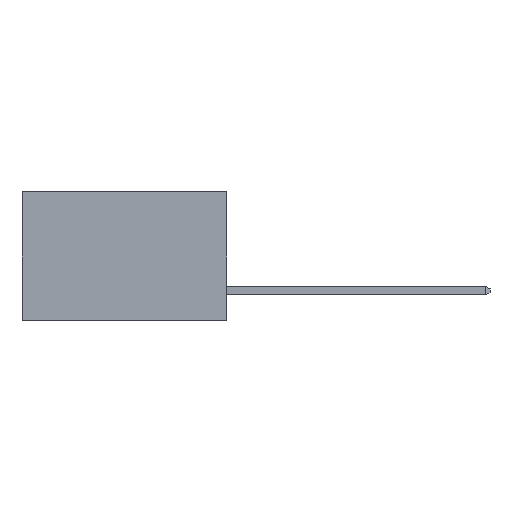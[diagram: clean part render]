
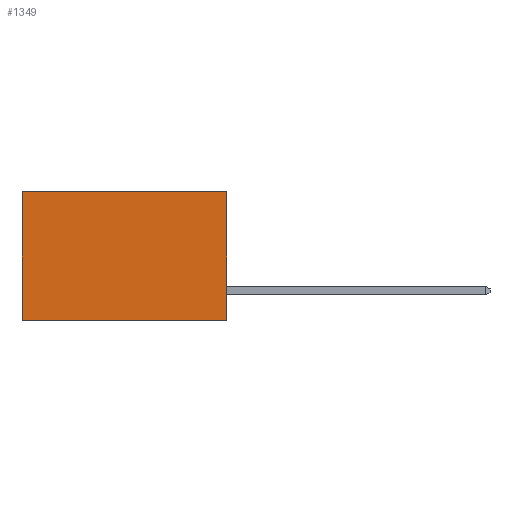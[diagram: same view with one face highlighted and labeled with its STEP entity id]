
A CAD part, left-side view. The second image highlights one B-rep face of the part: STEP entity #1349.
In plain terms, the highlighted planar face has unit normal (-1, 0, 0).
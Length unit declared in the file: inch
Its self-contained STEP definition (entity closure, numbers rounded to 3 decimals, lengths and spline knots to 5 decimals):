
#685 = VERTEX_POINT ( 'NONE', #7083 ) ;
#694 = DIRECTION ( 'NONE',  ( 0., 1., 0. ) ) ;
#1349 = ADVANCED_FACE ( 'NONE', ( #7775 ), #1897, .F. ) ;
#1603 = VERTEX_POINT ( 'NONE', #3541 ) ;
#1897 = PLANE ( 'NONE',  #5435 ) ;
#2203 = VERTEX_POINT ( 'NONE', #6520 ) ;
#2267 = DIRECTION ( 'NONE',  ( 0., 1., 0. ) ) ;
#2313 = CARTESIAN_POINT ( 'NONE',  ( 0.277, 0., 0. ) ) ;
#3097 = ORIENTED_EDGE ( 'NONE', *, *, #9133, .T. ) ;
#3155 = VECTOR ( 'NONE', #8713, 39.37008 ) ;
#3541 = CARTESIAN_POINT ( 'NONE',  ( 0.277, 0., -0.37 ) ) ;
#3729 = EDGE_LOOP ( 'NONE', ( #3097, #8240, #5666, #4572 ) ) ;
#3754 = VECTOR ( 'NONE', #694, 39.37008 ) ;
#4568 = LINE ( 'NONE', #7532, #7610 ) ;
#4572 = ORIENTED_EDGE ( 'NONE', *, *, #7996, .T. ) ;
#5223 = CARTESIAN_POINT ( 'NONE',  ( 0.277, 0., -0.37 ) ) ;
#5280 = VECTOR ( 'NONE', #2267, 39.37008 ) ;
#5435 = AXIS2_PLACEMENT_3D ( 'NONE', #7129, #5505, #9058 ) ;
#5505 = DIRECTION ( 'NONE',  ( 1., 0., 0. ) ) ;
#5666 = ORIENTED_EDGE ( 'NONE', *, *, #6993, .F. ) ;
#6520 = CARTESIAN_POINT ( 'NONE',  ( 0.277, 0.59, 0. ) ) ;
#6968 = CARTESIAN_POINT ( 'NONE',  ( 0.277, 0.59, -0.37 ) ) ;
#6993 = EDGE_CURVE ( 'NONE', #685, #1603, #8675, .T. ) ;
#7083 = CARTESIAN_POINT ( 'NONE',  ( 0.277, 0., 0. ) ) ;
#7129 = CARTESIAN_POINT ( 'NONE',  ( 0.277, 0., -0.37 ) ) ;
#7138 = LINE ( 'NONE', #2313, #5280 ) ;
#7306 = VERTEX_POINT ( 'NONE', #6968 ) ;
#7532 = CARTESIAN_POINT ( 'NONE',  ( 0.277, 0.59, -0.37 ) ) ;
#7610 = VECTOR ( 'NONE', #8661, 39.37008 ) ;
#7775 = FACE_OUTER_BOUND ( 'NONE', #3729, .T. ) ;
#7996 = EDGE_CURVE ( 'NONE', #685, #2203, #7138, .T. ) ;
#8240 = ORIENTED_EDGE ( 'NONE', *, *, #8955, .F. ) ;
#8661 = DIRECTION ( 'NONE',  ( 0., 0., -1. ) ) ;
#8675 = LINE ( 'NONE', #8728, #3155 ) ;
#8713 = DIRECTION ( 'NONE',  ( 0., 0., -1. ) ) ;
#8728 = CARTESIAN_POINT ( 'NONE',  ( 0.277, 0., -0.37 ) ) ;
#8955 = EDGE_CURVE ( 'NONE', #1603, #7306, #9214, .T. ) ;
#9058 = DIRECTION ( 'NONE',  ( 0., 0., -1. ) ) ;
#9133 = EDGE_CURVE ( 'NONE', #2203, #7306, #4568, .T. ) ;
#9214 = LINE ( 'NONE', #5223, #3754 ) ;
